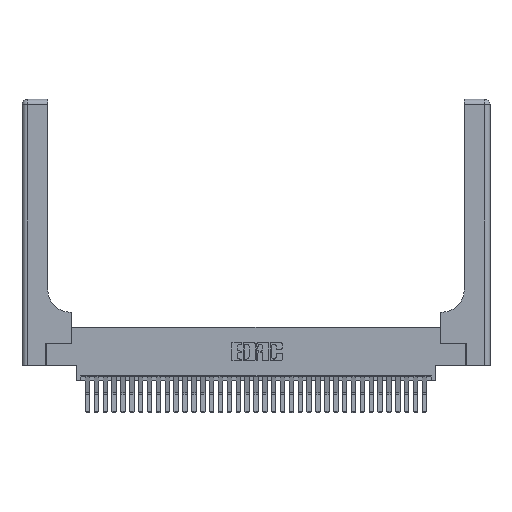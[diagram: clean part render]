
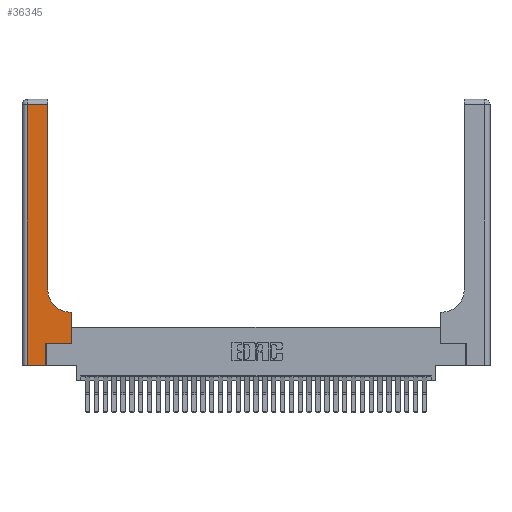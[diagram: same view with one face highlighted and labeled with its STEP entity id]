
A CAD part, top view. The second image highlights one B-rep face of the part: STEP entity #36345.
In plain terms, the highlighted planar face has unit normal (0, 0, 1).
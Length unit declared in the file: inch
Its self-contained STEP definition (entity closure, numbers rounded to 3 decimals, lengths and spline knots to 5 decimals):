
#228 = CARTESIAN_POINT ( 'NONE',  ( 0.2915, 2.94, 0.37 ) ) ;
#567 = ORIENTED_EDGE ( 'NONE', *, *, #24600, .T. ) ;
#636 = DIRECTION ( 'NONE',  ( 1., 0., 0. ) ) ;
#1840 = VECTOR ( 'NONE', #636, 39.37008 ) ;
#3286 = EDGE_LOOP ( 'NONE', ( #32251, #9813, #28355, #10158, #5850, #20395, #567, #22341, #28406 ) ) ;
#3944 = CARTESIAN_POINT ( 'NONE',  ( 0.5415, 0.85, 0.37 ) ) ;
#5850 = ORIENTED_EDGE ( 'NONE', *, *, #18421, .T. ) ;
#6111 = VERTEX_POINT ( 'NONE', #17670 ) ;
#6828 = DIRECTION ( 'NONE',  ( 1., 0., 0. ) ) ;
#7072 = CARTESIAN_POINT ( 'NONE',  ( 0.269, 0., 0.37 ) ) ;
#7364 = VECTOR ( 'NONE', #8809, 39.37008 ) ;
#7422 = CARTESIAN_POINT ( 'NONE',  ( 0.5415, 0.6, 0.37 ) ) ;
#7554 = CARTESIAN_POINT ( 'NONE',  ( 0.269, 0., 0.37 ) ) ;
#8206 = CARTESIAN_POINT ( 'NONE',  ( 0., 3., 0.37 ) ) ;
#8253 = LINE ( 'NONE', #33926, #7364 ) ;
#8275 = CARTESIAN_POINT ( 'NONE',  ( 0.2915, 0.6, 0.37 ) ) ;
#8809 = DIRECTION ( 'NONE',  ( 0., 1., 0. ) ) ;
#9813 = ORIENTED_EDGE ( 'NONE', *, *, #32294, .T. ) ;
#9928 = VECTOR ( 'NONE', #23953, 39.37008 ) ;
#10158 = ORIENTED_EDGE ( 'NONE', *, *, #26151, .T. ) ;
#10897 = LINE ( 'NONE', #13084, #31523 ) ;
#11062 = DIRECTION ( 'NONE',  ( -1., 0., 0. ) ) ;
#11136 = DIRECTION ( 'NONE',  ( -1., 0., 0. ) ) ;
#11499 = AXIS2_PLACEMENT_3D ( 'NONE', #3944, #23717, #6828 ) ;
#12683 = VERTEX_POINT ( 'NONE', #7554 ) ;
#13084 = CARTESIAN_POINT ( 'NONE',  ( 0., 0., 0.37 ) ) ;
#13365 = VECTOR ( 'NONE', #11136, 39.37008 ) ;
#13650 = EDGE_CURVE ( 'NONE', #23220, #6111, #28127, .T. ) ;
#14824 = EDGE_CURVE ( 'NONE', #33719, #33658, #28190, .T. ) ;
#14924 = CARTESIAN_POINT ( 'NONE',  ( 0.269, 0.25, 0.37 ) ) ;
#15002 = DIRECTION ( 'NONE',  ( 0., -1., 0. ) ) ;
#15120 = VECTOR ( 'NONE', #20678, 39.37008 ) ;
#15562 = LINE ( 'NONE', #33508, #31224 ) ;
#16864 = DIRECTION ( 'NONE',  ( -1., 0., 0. ) ) ;
#17670 = CARTESIAN_POINT ( 'NONE',  ( 0.06, 0., 0.37 ) ) ;
#18421 = EDGE_CURVE ( 'NONE', #12683, #26953, #28368, .T. ) ;
#18608 = VERTEX_POINT ( 'NONE', #24656 ) ;
#18969 = CARTESIAN_POINT ( 'NONE',  ( 0.5585, 0.6, 0.37 ) ) ;
#20395 = ORIENTED_EDGE ( 'NONE', *, *, #22280, .T. ) ;
#20678 = DIRECTION ( 'NONE',  ( 0., 1., 0. ) ) ;
#20770 = VECTOR ( 'NONE', #15002, 39.37008 ) ;
#22280 = EDGE_CURVE ( 'NONE', #26953, #18608, #24401, .T. ) ;
#22341 = ORIENTED_EDGE ( 'NONE', *, *, #14824, .T. ) ;
#22580 = CIRCLE ( 'NONE', #11499, 0.25 ) ;
#23220 = VERTEX_POINT ( 'NONE', #32870 ) ;
#23717 = DIRECTION ( 'NONE',  ( 0., 0., -1. ) ) ;
#23953 = DIRECTION ( 'NONE',  ( 0., 1., 0. ) ) ;
#24306 = DIRECTION ( 'NONE',  ( 1., 0., 0. ) ) ;
#24401 = LINE ( 'NONE', #14924, #1840 ) ;
#24600 = EDGE_CURVE ( 'NONE', #18608, #33719, #29902, .T. ) ;
#24656 = CARTESIAN_POINT ( 'NONE',  ( 0.5585, 0.25, 0.37 ) ) ;
#25425 = AXIS2_PLACEMENT_3D ( 'NONE', #8206, #27843, #11062 ) ;
#26151 = EDGE_CURVE ( 'NONE', #6111, #12683, #10897, .T. ) ;
#26224 = CARTESIAN_POINT ( 'NONE',  ( 0.5585, 0.25, 0.37 ) ) ;
#26953 = VERTEX_POINT ( 'NONE', #30365 ) ;
#27165 = VERTEX_POINT ( 'NONE', #28882 ) ;
#27843 = DIRECTION ( 'NONE',  ( 0., 0., -1. ) ) ;
#27888 = FACE_OUTER_BOUND ( 'NONE', #3286, .T. ) ;
#28127 = LINE ( 'NONE', #28860, #20770 ) ;
#28190 = LINE ( 'NONE', #8275, #13365 ) ;
#28286 = EDGE_CURVE ( 'NONE', #27165, #33988, #8253, .T. ) ;
#28355 = ORIENTED_EDGE ( 'NONE', *, *, #13650, .T. ) ;
#28368 = LINE ( 'NONE', #7072, #9928 ) ;
#28406 = ORIENTED_EDGE ( 'NONE', *, *, #31227, .T. ) ;
#28860 = CARTESIAN_POINT ( 'NONE',  ( 0.06, 3., 0.37 ) ) ;
#28882 = CARTESIAN_POINT ( 'NONE',  ( 0.2915, 0.85, 0.37 ) ) ;
#29902 = LINE ( 'NONE', #26224, #15120 ) ;
#30365 = CARTESIAN_POINT ( 'NONE',  ( 0.269, 0.25, 0.37 ) ) ;
#31224 = VECTOR ( 'NONE', #16864, 39.37008 ) ;
#31227 = EDGE_CURVE ( 'NONE', #33658, #27165, #22580, .T. ) ;
#31523 = VECTOR ( 'NONE', #24306, 39.37008 ) ;
#32251 = ORIENTED_EDGE ( 'NONE', *, *, #28286, .T. ) ;
#32294 = EDGE_CURVE ( 'NONE', #33988, #23220, #15562, .T. ) ;
#32870 = CARTESIAN_POINT ( 'NONE',  ( 0.06, 2.94, 0.37 ) ) ;
#33508 = CARTESIAN_POINT ( 'NONE',  ( 0., 2.94, 0.37 ) ) ;
#33658 = VERTEX_POINT ( 'NONE', #7422 ) ;
#33719 = VERTEX_POINT ( 'NONE', #18969 ) ;
#33926 = CARTESIAN_POINT ( 'NONE',  ( 0.2915, 3., 0.37 ) ) ;
#33988 = VERTEX_POINT ( 'NONE', #228 ) ;
#35960 = PLANE ( 'NONE',  #25425 ) ;
#36345 = ADVANCED_FACE ( 'NONE', ( #27888 ), #35960, .F. ) ;
